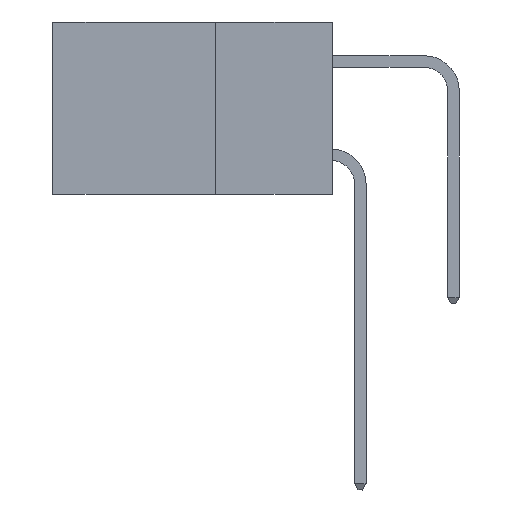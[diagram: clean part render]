
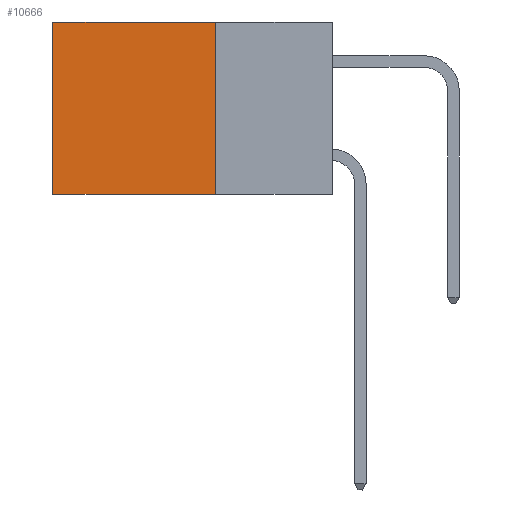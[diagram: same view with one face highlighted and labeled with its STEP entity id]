
A CAD part, left-side view. The second image highlights one B-rep face of the part: STEP entity #10666.
In plain terms, the highlighted planar face has unit normal (-1, 0, 0).
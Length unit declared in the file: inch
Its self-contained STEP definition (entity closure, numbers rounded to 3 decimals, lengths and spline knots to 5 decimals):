
#721 = CARTESIAN_POINT ( 'NONE',  ( 0.298, 0.25, -0.37 ) ) ;
#948 = ORIENTED_EDGE ( 'NONE', *, *, #24528, .F. ) ;
#965 = ORIENTED_EDGE ( 'NONE', *, *, #20484, .T. ) ;
#1944 = LINE ( 'NONE', #5420, #22006 ) ;
#4275 = EDGE_CURVE ( 'NONE', #13400, #19229, #23518, .T. ) ;
#5420 = CARTESIAN_POINT ( 'NONE',  ( 0.298, 0.25, 0. ) ) ;
#6085 = DIRECTION ( 'NONE',  ( 0., 0., -1. ) ) ;
#7520 = CARTESIAN_POINT ( 'NONE',  ( 0.298, 0.6, -0.37 ) ) ;
#8220 = EDGE_LOOP ( 'NONE', ( #965, #948, #17638, #24081 ) ) ;
#8804 = CARTESIAN_POINT ( 'NONE',  ( 0.298, 0.6, 0. ) ) ;
#8877 = VECTOR ( 'NONE', #25973, 39.37008 ) ;
#10041 = CARTESIAN_POINT ( 'NONE',  ( 0.298, 0.25, 0. ) ) ;
#10666 = ADVANCED_FACE ( 'NONE', ( #21221 ), #11768, .F. ) ;
#11632 = AXIS2_PLACEMENT_3D ( 'NONE', #29927, #14349, #32648 ) ;
#11768 = PLANE ( 'NONE',  #11632 ) ;
#13250 = VECTOR ( 'NONE', #32170, 39.37008 ) ;
#13400 = VERTEX_POINT ( 'NONE', #30566 ) ;
#14349 = DIRECTION ( 'NONE',  ( 1., 0., 0. ) ) ;
#17043 = EDGE_CURVE ( 'NONE', #13400, #29035, #1944, .T. ) ;
#17638 = ORIENTED_EDGE ( 'NONE', *, *, #4275, .F. ) ;
#19157 = CARTESIAN_POINT ( 'NONE',  ( 0.298, 0.6, 0. ) ) ;
#19229 = VERTEX_POINT ( 'NONE', #721 ) ;
#20248 = VERTEX_POINT ( 'NONE', #7520 ) ;
#20484 = EDGE_CURVE ( 'NONE', #29035, #20248, #26413, .T. ) ;
#21221 = FACE_OUTER_BOUND ( 'NONE', #8220, .T. ) ;
#22006 = VECTOR ( 'NONE', #26349, 39.37008 ) ;
#22676 = VECTOR ( 'NONE', #6085, 39.37008 ) ;
#23518 = LINE ( 'NONE', #10041, #22676 ) ;
#24081 = ORIENTED_EDGE ( 'NONE', *, *, #17043, .T. ) ;
#24528 = EDGE_CURVE ( 'NONE', #19229, #20248, #29739, .T. ) ;
#25973 = DIRECTION ( 'NONE',  ( 0., 1., 0. ) ) ;
#26349 = DIRECTION ( 'NONE',  ( 0., 1., 0. ) ) ;
#26413 = LINE ( 'NONE', #19157, #13250 ) ;
#29035 = VERTEX_POINT ( 'NONE', #8804 ) ;
#29739 = LINE ( 'NONE', #31058, #8877 ) ;
#29927 = CARTESIAN_POINT ( 'NONE',  ( 0.298, 0.25, 0. ) ) ;
#30566 = CARTESIAN_POINT ( 'NONE',  ( 0.298, 0.25, 0. ) ) ;
#31058 = CARTESIAN_POINT ( 'NONE',  ( 0.298, 0.25, -0.37 ) ) ;
#32170 = DIRECTION ( 'NONE',  ( 0., 0., -1. ) ) ;
#32648 = DIRECTION ( 'NONE',  ( 0., 0., -1. ) ) ;
